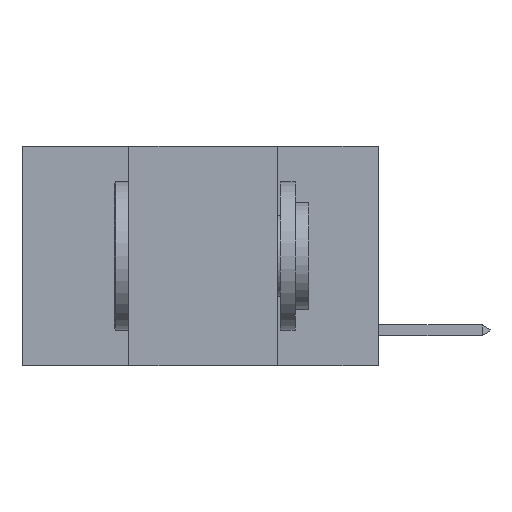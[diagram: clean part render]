
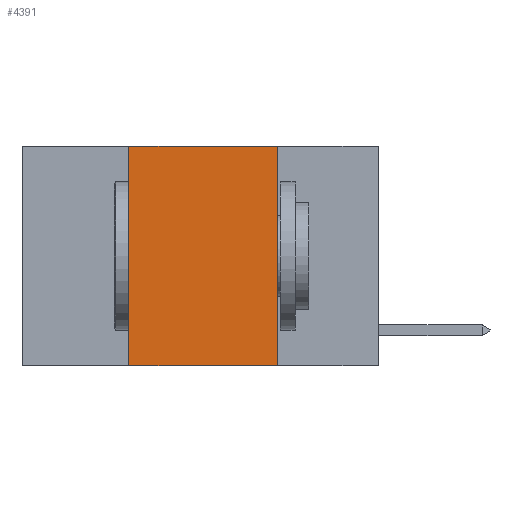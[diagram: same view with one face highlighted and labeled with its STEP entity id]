
A CAD part, left-side view. The second image highlights one B-rep face of the part: STEP entity #4391.
In plain terms, the highlighted planar face has unit normal (-1, 0, 0).
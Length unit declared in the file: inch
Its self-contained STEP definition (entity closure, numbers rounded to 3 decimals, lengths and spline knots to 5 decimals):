
#248 = DIRECTION ( 'NONE',  ( 0., -1., 0. ) ) ;
#412 = CARTESIAN_POINT ( 'NONE',  ( 0., 0.42, 0. ) ) ;
#1350 = VERTEX_POINT ( 'NONE', #9767 ) ;
#1397 = ORIENTED_EDGE ( 'NONE', *, *, #6594, .F. ) ;
#1987 = LINE ( 'NONE', #3623, #9304 ) ;
#2438 = CARTESIAN_POINT ( 'NONE',  ( 0., 0.17, 0. ) ) ;
#2846 = VERTEX_POINT ( 'NONE', #412 ) ;
#3003 = EDGE_CURVE ( 'NONE', #1350, #2846, #1987, .T. ) ;
#3623 = CARTESIAN_POINT ( 'NONE',  ( 0., 0.42, 0. ) ) ;
#4391 = ADVANCED_FACE ( 'NONE', ( #17009 ), #16911, .F. ) ;
#4547 = ORIENTED_EDGE ( 'NONE', *, *, #3003, .F. ) ;
#4820 = CARTESIAN_POINT ( 'NONE',  ( 0., 0.17, -0.37 ) ) ;
#5818 = VERTEX_POINT ( 'NONE', #10589 ) ;
#6572 = DIRECTION ( 'NONE',  ( 0., 0., 1. ) ) ;
#6594 = EDGE_CURVE ( 'NONE', #5818, #11603, #15397, .T. ) ;
#6663 = ORIENTED_EDGE ( 'NONE', *, *, #10767, .T. ) ;
#6750 = DIRECTION ( 'NONE',  ( 1., 0., 0. ) ) ;
#6786 = AXIS2_PLACEMENT_3D ( 'NONE', #8631, #6750, #12495 ) ;
#7635 = LINE ( 'NONE', #17827, #10672 ) ;
#7871 = DIRECTION ( 'NONE',  ( 0., 0., -1. ) ) ;
#8416 = VECTOR ( 'NONE', #7871, 39.37008 ) ;
#8494 = VECTOR ( 'NONE', #248, 39.37008 ) ;
#8631 = CARTESIAN_POINT ( 'NONE',  ( 0., 0.6, 0. ) ) ;
#9304 = VECTOR ( 'NONE', #6572, 39.37008 ) ;
#9386 = EDGE_CURVE ( 'NONE', #2846, #5818, #11673, .T. ) ;
#9767 = CARTESIAN_POINT ( 'NONE',  ( 0., 0.42, -0.37 ) ) ;
#10589 = CARTESIAN_POINT ( 'NONE',  ( 0., 0.17, 0. ) ) ;
#10672 = VECTOR ( 'NONE', #13191, 39.37008 ) ;
#10767 = EDGE_CURVE ( 'NONE', #1350, #11603, #7635, .T. ) ;
#11603 = VERTEX_POINT ( 'NONE', #4820 ) ;
#11673 = LINE ( 'NONE', #14583, #8494 ) ;
#12495 = DIRECTION ( 'NONE',  ( 0., 0., -1. ) ) ;
#13191 = DIRECTION ( 'NONE',  ( 0., -1., 0. ) ) ;
#14583 = CARTESIAN_POINT ( 'NONE',  ( 0., 0.6, 0. ) ) ;
#15397 = LINE ( 'NONE', #2438, #8416 ) ;
#16911 = PLANE ( 'NONE',  #6786 ) ;
#17009 = FACE_OUTER_BOUND ( 'NONE', #17422, .T. ) ;
#17422 = EDGE_LOOP ( 'NONE', ( #1397, #18008, #4547, #6663 ) ) ;
#17827 = CARTESIAN_POINT ( 'NONE',  ( 0., 0.6, -0.37 ) ) ;
#18008 = ORIENTED_EDGE ( 'NONE', *, *, #9386, .F. ) ;
